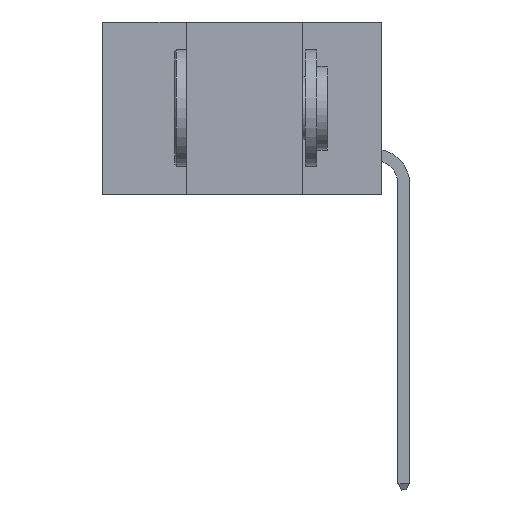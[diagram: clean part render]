
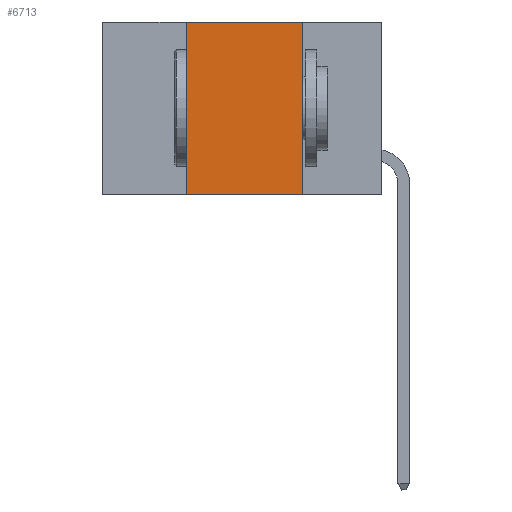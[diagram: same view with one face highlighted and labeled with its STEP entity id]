
A CAD part, left-side view. The second image highlights one B-rep face of the part: STEP entity #6713.
In plain terms, the highlighted planar face has unit normal (-1, 0, 0).
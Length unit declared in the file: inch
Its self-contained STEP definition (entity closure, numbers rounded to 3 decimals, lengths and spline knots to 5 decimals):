
#722 = VERTEX_POINT ( 'NONE', #18109 ) ;
#1209 = ORIENTED_EDGE ( 'NONE', *, *, #3914, .F. ) ;
#3914 = EDGE_CURVE ( 'NONE', #40285, #36182, #32356, .T. ) ;
#6584 = ORIENTED_EDGE ( 'NONE', *, *, #39811, .F. ) ;
#6713 = ADVANCED_FACE ( 'NONE', ( #11327 ), #30136, .F. ) ;
#7508 = EDGE_CURVE ( 'NONE', #23736, #722, #31914, .T. ) ;
#7830 = CARTESIAN_POINT ( 'NONE',  ( 0., 0.17, 0. ) ) ;
#8375 = CARTESIAN_POINT ( 'NONE',  ( 0., 0.17, 0. ) ) ;
#9152 = VECTOR ( 'NONE', #11429, 39.37008 ) ;
#9931 = EDGE_LOOP ( 'NONE', ( #10389, #6584, #1209, #39038 ) ) ;
#10389 = ORIENTED_EDGE ( 'NONE', *, *, #7508, .F. ) ;
#11327 = FACE_OUTER_BOUND ( 'NONE', #9931, .T. ) ;
#11429 = DIRECTION ( 'NONE',  ( 0., -1., 0. ) ) ;
#15058 = CARTESIAN_POINT ( 'NONE',  ( 0., 0.6, -0.37 ) ) ;
#15152 = CARTESIAN_POINT ( 'NONE',  ( 0., 0.6, 0. ) ) ;
#17179 = DIRECTION ( 'NONE',  ( 1., 0., 0. ) ) ;
#18109 = CARTESIAN_POINT ( 'NONE',  ( 0., 0.17, -0.37 ) ) ;
#18233 = CARTESIAN_POINT ( 'NONE',  ( 0., 0.42, -0.37 ) ) ;
#20247 = CARTESIAN_POINT ( 'NONE',  ( 0., 0.6, 0. ) ) ;
#23032 = VECTOR ( 'NONE', #38325, 39.37008 ) ;
#23736 = VERTEX_POINT ( 'NONE', #8375 ) ;
#25160 = LINE ( 'NONE', #15152, #23032 ) ;
#25868 = DIRECTION ( 'NONE',  ( 0., 0., 1. ) ) ;
#28366 = LINE ( 'NONE', #15058, #9152 ) ;
#30136 = PLANE ( 'NONE',  #33079 ) ;
#31181 = DIRECTION ( 'NONE',  ( 0., 0., -1. ) ) ;
#31914 = LINE ( 'NONE', #7830, #34460 ) ;
#32356 = LINE ( 'NONE', #41640, #39077 ) ;
#33079 = AXIS2_PLACEMENT_3D ( 'NONE', #20247, #17179, #40374 ) ;
#34460 = VECTOR ( 'NONE', #31181, 39.37008 ) ;
#36182 = VERTEX_POINT ( 'NONE', #42488 ) ;
#38325 = DIRECTION ( 'NONE',  ( 0., -1., 0. ) ) ;
#38984 = EDGE_CURVE ( 'NONE', #40285, #722, #28366, .T. ) ;
#39038 = ORIENTED_EDGE ( 'NONE', *, *, #38984, .T. ) ;
#39077 = VECTOR ( 'NONE', #25868, 39.37008 ) ;
#39811 = EDGE_CURVE ( 'NONE', #36182, #23736, #25160, .T. ) ;
#40285 = VERTEX_POINT ( 'NONE', #18233 ) ;
#40374 = DIRECTION ( 'NONE',  ( 0., 0., -1. ) ) ;
#41640 = CARTESIAN_POINT ( 'NONE',  ( 0., 0.42, 0. ) ) ;
#42488 = CARTESIAN_POINT ( 'NONE',  ( 0., 0.42, 0. ) ) ;
